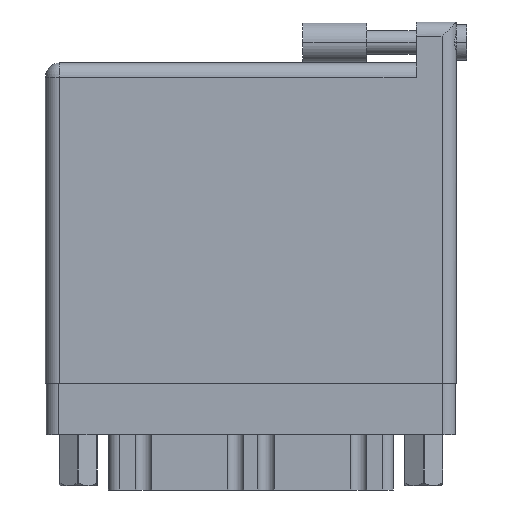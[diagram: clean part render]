
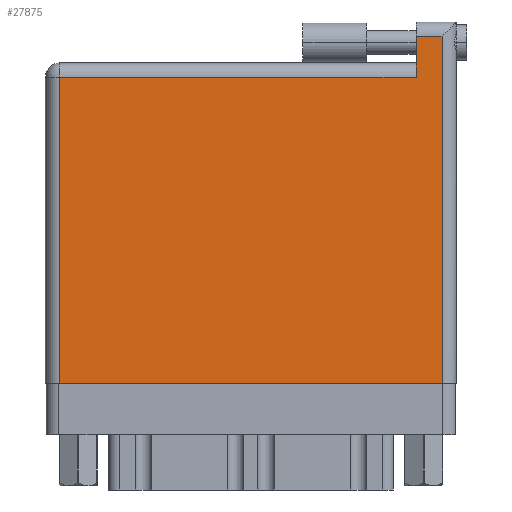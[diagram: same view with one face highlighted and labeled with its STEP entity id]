
A CAD part, front view. The second image highlights one B-rep face of the part: STEP entity #27875.
In plain terms, the highlighted face is planar.
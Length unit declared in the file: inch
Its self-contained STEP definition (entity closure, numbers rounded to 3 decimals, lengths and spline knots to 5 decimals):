
#279 = CARTESIAN_POINT ( 'NONE',  ( 1.811, 1.496, 0. ) ) ;
#2412 = CARTESIAN_POINT ( 'NONE',  ( 1.811, 1.766, 0. ) ) ;
#3675 = CARTESIAN_POINT ( 'NONE',  ( 1.938, 1.696, 0. ) ) ;
#3757 = VERTEX_POINT ( 'NONE', #3675 ) ;
#3826 = ORIENTED_EDGE ( 'NONE', *, *, #43535, .T. ) ;
#4853 = LINE ( 'NONE', #31203, #45801 ) ;
#5059 = LINE ( 'NONE', #26882, #39708 ) ;
#5644 = VERTEX_POINT ( 'NONE', #279 ) ;
#6478 = VECTOR ( 'NONE', #32136, 39.37008 ) ;
#6731 = VERTEX_POINT ( 'NONE', #18774 ) ;
#6963 = EDGE_CURVE ( 'NONE', #32551, #41586, #4853, .T. ) ;
#7942 = DIRECTION ( 'NONE',  ( 0., 1., 0. ) ) ;
#8993 = VECTOR ( 'NONE', #43319, 39.37008 ) ;
#10672 = VECTOR ( 'NONE', #20532, 39.37008 ) ;
#11447 = DIRECTION ( 'NONE',  ( -1., 0., 0. ) ) ;
#14027 = ORIENTED_EDGE ( 'NONE', *, *, #44830, .T. ) ;
#14446 = ORIENTED_EDGE ( 'NONE', *, *, #20521, .T. ) ;
#14458 = ORIENTED_EDGE ( 'NONE', *, *, #45654, .T. ) ;
#16941 = CARTESIAN_POINT ( 'NONE',  ( 0.07, 0., 0. ) ) ;
#18774 = CARTESIAN_POINT ( 'NONE',  ( 0.07, 1.496, 0. ) ) ;
#19625 = ORIENTED_EDGE ( 'NONE', *, *, #42319, .T. ) ;
#19828 = VECTOR ( 'NONE', #11447, 39.37008 ) ;
#20521 = EDGE_CURVE ( 'NONE', #6731, #32551, #35635, .T. ) ;
#20532 = DIRECTION ( 'NONE',  ( 0., -1., 0. ) ) ;
#22177 = CARTESIAN_POINT ( 'NONE',  ( 0., 1.566, 0. ) ) ;
#22938 = CARTESIAN_POINT ( 'NONE',  ( 0., 1.496, 0. ) ) ;
#25363 = CARTESIAN_POINT ( 'NONE',  ( 0., 1.696, 0. ) ) ;
#26006 = AXIS2_PLACEMENT_3D ( 'NONE', #22177, #36803, #43261 ) ;
#26882 = CARTESIAN_POINT ( 'NONE',  ( 1.938, 1.766, 0. ) ) ;
#27875 = ADVANCED_FACE ( 'NONE', ( #28898 ), #28672, .F. ) ;
#28672 = PLANE ( 'NONE',  #26006 ) ;
#28898 = FACE_OUTER_BOUND ( 'NONE', #33716, .T. ) ;
#30839 = LINE ( 'NONE', #22938, #19828 ) ;
#31203 = CARTESIAN_POINT ( 'NONE',  ( 0., 0., 0. ) ) ;
#32136 = DIRECTION ( 'NONE',  ( 0., -1., 0. ) ) ;
#32551 = VERTEX_POINT ( 'NONE', #38272 ) ;
#33716 = EDGE_LOOP ( 'NONE', ( #43428, #14027, #3826, #19625, #14458, #14446 ) ) ;
#35635 = LINE ( 'NONE', #16941, #10672 ) ;
#36402 = LINE ( 'NONE', #25363, #8993 ) ;
#36803 = DIRECTION ( 'NONE',  ( 0., 0., -1. ) ) ;
#37370 = CARTESIAN_POINT ( 'NONE',  ( 1.811, 1.696, 0. ) ) ;
#38272 = CARTESIAN_POINT ( 'NONE',  ( 0.07, 0., 0. ) ) ;
#39708 = VECTOR ( 'NONE', #7942, 39.37008 ) ;
#41274 = DIRECTION ( 'NONE',  ( 1., 0., 0. ) ) ;
#41586 = VERTEX_POINT ( 'NONE', #42381 ) ;
#42319 = EDGE_CURVE ( 'NONE', #45073, #5644, #42908, .T. ) ;
#42381 = CARTESIAN_POINT ( 'NONE',  ( 1.938, 0., 0. ) ) ;
#42908 = LINE ( 'NONE', #2412, #6478 ) ;
#43261 = DIRECTION ( 'NONE',  ( -1., 0., 0. ) ) ;
#43319 = DIRECTION ( 'NONE',  ( -1., 0., 0. ) ) ;
#43428 = ORIENTED_EDGE ( 'NONE', *, *, #6963, .T. ) ;
#43535 = EDGE_CURVE ( 'NONE', #3757, #45073, #36402, .T. ) ;
#44830 = EDGE_CURVE ( 'NONE', #41586, #3757, #5059, .T. ) ;
#45073 = VERTEX_POINT ( 'NONE', #37370 ) ;
#45654 = EDGE_CURVE ( 'NONE', #5644, #6731, #30839, .T. ) ;
#45801 = VECTOR ( 'NONE', #41274, 39.37008 ) ;
